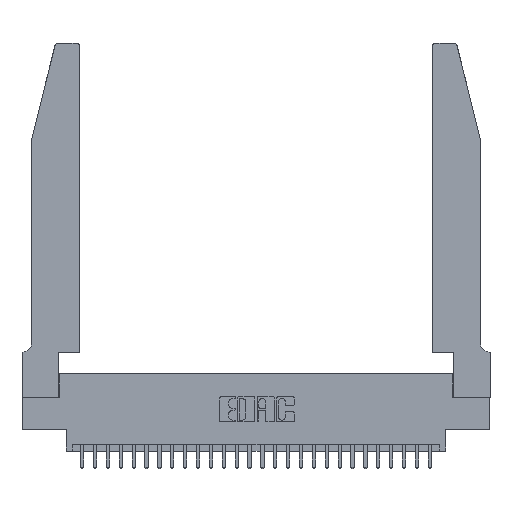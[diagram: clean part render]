
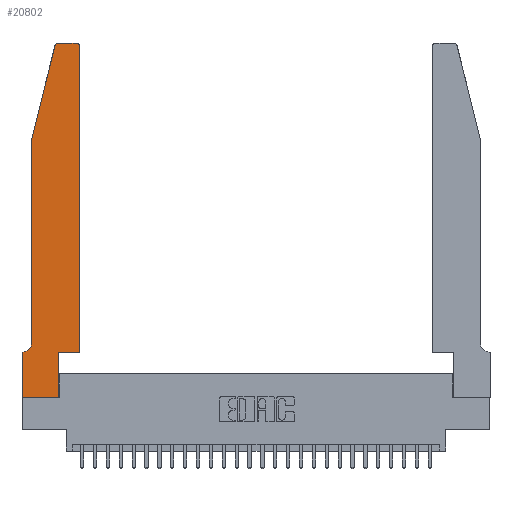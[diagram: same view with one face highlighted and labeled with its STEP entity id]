
A CAD part, top view. The second image highlights one B-rep face of the part: STEP entity #20802.
In plain terms, the highlighted planar face has unit normal (0, 0, 1).
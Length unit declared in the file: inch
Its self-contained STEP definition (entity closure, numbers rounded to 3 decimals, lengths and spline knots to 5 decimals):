
#122 = LINE ( 'NONE', #27394, #23245 ) ;
#247 = VERTEX_POINT ( 'NONE', #2696 ) ;
#252 = VECTOR ( 'NONE', #21625, 39.37008 ) ;
#540 = ORIENTED_EDGE ( 'NONE', *, *, #13270, .T. ) ;
#703 = VECTOR ( 'NONE', #28183, 39.37008 ) ;
#743 = DIRECTION ( 'NONE',  ( 1., 0., 0. ) ) ;
#1206 = EDGE_CURVE ( 'NONE', #5012, #4261, #11346, .T. ) ;
#1912 = EDGE_LOOP ( 'NONE', ( #15270, #18073, #6907, #21560, #12457, #14254, #6087, #20026, #26138, #14355, #540, #13436 ) ) ;
#2497 = VECTOR ( 'NONE', #12302, 39.37008 ) ;
#2696 = CARTESIAN_POINT ( 'NONE',  ( 0.0055, 0.35, 0.37 ) ) ;
#2794 = CARTESIAN_POINT ( 'NONE',  ( 0.2865, 0.35, 0.37 ) ) ;
#2939 = CARTESIAN_POINT ( 'NONE',  ( 0.4205, 2.75, 0.37 ) ) ;
#3119 = EDGE_CURVE ( 'NONE', #20121, #5549, #122, .T. ) ;
#3608 = VERTEX_POINT ( 'NONE', #24890 ) ;
#3662 = CARTESIAN_POINT ( 'NONE',  ( 0.2865, 0.35, 0.37 ) ) ;
#4008 = VERTEX_POINT ( 'NONE', #8683 ) ;
#4251 = VECTOR ( 'NONE', #14341, 39.37008 ) ;
#4261 = VERTEX_POINT ( 'NONE', #2939 ) ;
#4366 = LINE ( 'NONE', #10315, #26513 ) ;
#4588 = DIRECTION ( 'NONE',  ( 0., 0., 1. ) ) ;
#4739 = CARTESIAN_POINT ( 'NONE',  ( 0.0755, 2., 0.37 ) ) ;
#5012 = VERTEX_POINT ( 'NONE', #23239 ) ;
#5266 = VERTEX_POINT ( 'NONE', #8618 ) ;
#5359 = CARTESIAN_POINT ( 'NONE',  ( 0.4505, 0.35, 0.37 ) ) ;
#5549 = VERTEX_POINT ( 'NONE', #6209 ) ;
#6087 = ORIENTED_EDGE ( 'NONE', *, *, #25156, .T. ) ;
#6088 = EDGE_CURVE ( 'NONE', #4008, #20451, #25430, .T. ) ;
#6159 = CARTESIAN_POINT ( 'NONE',  ( 0.284, 2.72, 0.37 ) ) ;
#6182 = LINE ( 'NONE', #26018, #703 ) ;
#6209 = CARTESIAN_POINT ( 'NONE',  ( 0.2865, 0., 0.37 ) ) ;
#6240 = VECTOR ( 'NONE', #9450, 39.37008 ) ;
#6542 = AXIS2_PLACEMENT_3D ( 'NONE', #8299, #23681, #10567 ) ;
#6907 = ORIENTED_EDGE ( 'NONE', *, *, #6088, .T. ) ;
#7152 = CIRCLE ( 'NONE', #6542, 0.07 ) ;
#7520 = DIRECTION ( 'NONE',  ( -1., 0., 0. ) ) ;
#8091 = AXIS2_PLACEMENT_3D ( 'NONE', #22349, #22448, #22237 ) ;
#8299 = CARTESIAN_POINT ( 'NONE',  ( 0.0055, 0.42, 0.37 ) ) ;
#8431 = DIRECTION ( 'NONE',  ( 1., 0., 0. ) ) ;
#8618 = CARTESIAN_POINT ( 'NONE',  ( 0.284, 2.75, 0.37 ) ) ;
#8683 = CARTESIAN_POINT ( 'NONE',  ( 0.25487, 2.72718, 0.37 ) ) ;
#9450 = DIRECTION ( 'NONE',  ( 0., 1., 0. ) ) ;
#9504 = EDGE_CURVE ( 'NONE', #18347, #3608, #21362, .T. ) ;
#9903 = LINE ( 'NONE', #4739, #15844 ) ;
#10109 = CARTESIAN_POINT ( 'NONE',  ( 0.0755, 0.42, 0.37 ) ) ;
#10315 = CARTESIAN_POINT ( 'NONE',  ( 0., 0., 0.37 ) ) ;
#10567 = DIRECTION ( 'NONE',  ( -1., 0., 0. ) ) ;
#11201 = EDGE_CURVE ( 'NONE', #20451, #19003, #9903, .T. ) ;
#11301 = AXIS2_PLACEMENT_3D ( 'NONE', #28765, #4588, #20231 ) ;
#11346 = CIRCLE ( 'NONE', #8091, 0.03 ) ;
#12302 = DIRECTION ( 'NONE',  ( -0.239, -0.971, 0. ) ) ;
#12359 = LINE ( 'NONE', #21113, #16858 ) ;
#12457 = ORIENTED_EDGE ( 'NONE', *, *, #19171, .T. ) ;
#12570 = DIRECTION ( 'NONE',  ( 0., -1., 0. ) ) ;
#13270 = EDGE_CURVE ( 'NONE', #3608, #5012, #22485, .T. ) ;
#13436 = ORIENTED_EDGE ( 'NONE', *, *, #1206, .T. ) ;
#14235 = EDGE_CURVE ( 'NONE', #4261, #5266, #12359, .T. ) ;
#14254 = ORIENTED_EDGE ( 'NONE', *, *, #25773, .T. ) ;
#14341 = DIRECTION ( 'NONE',  ( 1., 0., 0. ) ) ;
#14355 = ORIENTED_EDGE ( 'NONE', *, *, #9504, .T. ) ;
#15270 = ORIENTED_EDGE ( 'NONE', *, *, #14235, .T. ) ;
#15844 = VECTOR ( 'NONE', #24653, 39.37008 ) ;
#15917 = FACE_OUTER_BOUND ( 'NONE', #1912, .T. ) ;
#16858 = VECTOR ( 'NONE', #7520, 39.37008 ) ;
#18047 = PLANE ( 'NONE',  #11301 ) ;
#18073 = ORIENTED_EDGE ( 'NONE', *, *, #22430, .T. ) ;
#18298 = LINE ( 'NONE', #3662, #252 ) ;
#18347 = VERTEX_POINT ( 'NONE', #2794 ) ;
#19003 = VERTEX_POINT ( 'NONE', #10109 ) ;
#19171 = EDGE_CURVE ( 'NONE', #19003, #247, #7152, .T. ) ;
#19180 = EDGE_CURVE ( 'NONE', #5549, #18347, #18298, .T. ) ;
#19209 = CIRCLE ( 'NONE', #25197, 0.03 ) ;
#20026 = ORIENTED_EDGE ( 'NONE', *, *, #3119, .T. ) ;
#20121 = VERTEX_POINT ( 'NONE', #24477 ) ;
#20231 = DIRECTION ( 'NONE',  ( 1., 0., 0. ) ) ;
#20451 = VERTEX_POINT ( 'NONE', #27670 ) ;
#20475 = CARTESIAN_POINT ( 'NONE',  ( 0.4505, 0.35, 0.37 ) ) ;
#20802 = ADVANCED_FACE ( 'NONE', ( #15917 ), #18047, .T. ) ;
#21113 = CARTESIAN_POINT ( 'NONE',  ( 0.2605, 2.75, 0.37 ) ) ;
#21362 = LINE ( 'NONE', #5359, #4251 ) ;
#21560 = ORIENTED_EDGE ( 'NONE', *, *, #11201, .T. ) ;
#21625 = DIRECTION ( 'NONE',  ( 0., 1., 0. ) ) ;
#21657 = DIRECTION ( 'NONE',  ( 0., 0., 1. ) ) ;
#22237 = DIRECTION ( 'NONE',  ( 1., 0., 0. ) ) ;
#22349 = CARTESIAN_POINT ( 'NONE',  ( 0.4205, 2.72, 0.37 ) ) ;
#22430 = EDGE_CURVE ( 'NONE', #5266, #4008, #19209, .T. ) ;
#22448 = DIRECTION ( 'NONE',  ( 0., 0., 1. ) ) ;
#22485 = LINE ( 'NONE', #20475, #6240 ) ;
#23163 = CARTESIAN_POINT ( 'NONE',  ( 0.0755, 2., 0.37 ) ) ;
#23239 = CARTESIAN_POINT ( 'NONE',  ( 0.4505, 2.72, 0.37 ) ) ;
#23245 = VECTOR ( 'NONE', #743, 39.37008 ) ;
#23681 = DIRECTION ( 'NONE',  ( 0., 0., -1. ) ) ;
#24477 = CARTESIAN_POINT ( 'NONE',  ( 0., 0., 0.37 ) ) ;
#24653 = DIRECTION ( 'NONE',  ( 0., -1., 0. ) ) ;
#24890 = CARTESIAN_POINT ( 'NONE',  ( 0.4505, 0.35, 0.37 ) ) ;
#25156 = EDGE_CURVE ( 'NONE', #26363, #20121, #4366, .T. ) ;
#25197 = AXIS2_PLACEMENT_3D ( 'NONE', #6159, #21657, #8431 ) ;
#25430 = LINE ( 'NONE', #23163, #2497 ) ;
#25773 = EDGE_CURVE ( 'NONE', #247, #26363, #6182, .T. ) ;
#26018 = CARTESIAN_POINT ( 'NONE',  ( 0.0755, 0.35, 0.37 ) ) ;
#26138 = ORIENTED_EDGE ( 'NONE', *, *, #19180, .T. ) ;
#26363 = VERTEX_POINT ( 'NONE', #27878 ) ;
#26513 = VECTOR ( 'NONE', #12570, 39.37008 ) ;
#27394 = CARTESIAN_POINT ( 'NONE',  ( 0., 0., 0.37 ) ) ;
#27670 = CARTESIAN_POINT ( 'NONE',  ( 0.0755, 2., 0.37 ) ) ;
#27878 = CARTESIAN_POINT ( 'NONE',  ( 0., 0.35, 0.37 ) ) ;
#28183 = DIRECTION ( 'NONE',  ( -1., 0., 0. ) ) ;
#28765 = CARTESIAN_POINT ( 'NONE',  ( 0., 0.35, 0.37 ) ) ;
